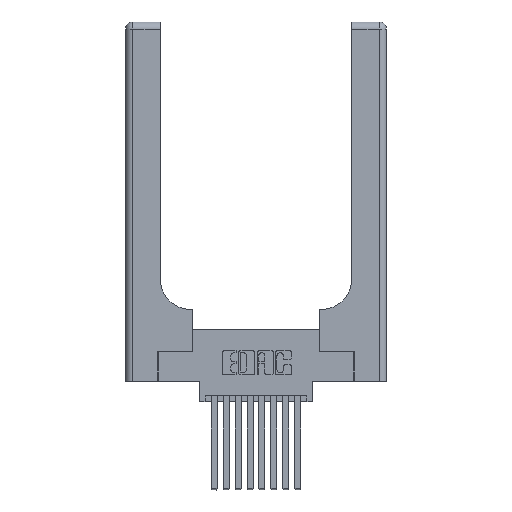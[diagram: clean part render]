
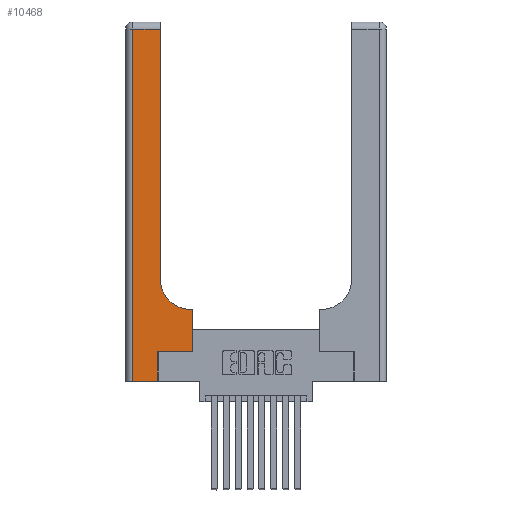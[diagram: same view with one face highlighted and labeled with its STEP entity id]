
A CAD part, top view. The second image highlights one B-rep face of the part: STEP entity #10468.
In plain terms, the highlighted planar face has unit normal (0, 0, 1).
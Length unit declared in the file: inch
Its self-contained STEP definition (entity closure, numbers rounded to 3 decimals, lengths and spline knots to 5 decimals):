
#297 = DIRECTION ( 'NONE',  ( -1., 0., 0. ) ) ;
#305 = ORIENTED_EDGE ( 'NONE', *, *, #3835, .T. ) ;
#359 = VERTEX_POINT ( 'NONE', #2186 ) ;
#690 = VECTOR ( 'NONE', #14108, 39.37008 ) ;
#743 = CARTESIAN_POINT ( 'NONE',  ( 0.06, 3., 0.37 ) ) ;
#803 = EDGE_LOOP ( 'NONE', ( #5306, #8881, #305, #12754, #1064, #12064, #5554, #12509, #13203 ) ) ;
#893 = DIRECTION ( 'NONE',  ( 0., 0., -1. ) ) ;
#1064 = ORIENTED_EDGE ( 'NONE', *, *, #12910, .T. ) ;
#1365 = VERTEX_POINT ( 'NONE', #3940 ) ;
#1384 = DIRECTION ( 'NONE',  ( 1., 0., 0. ) ) ;
#1552 = LINE ( 'NONE', #8978, #8720 ) ;
#1645 = CIRCLE ( 'NONE', #3491, 0.25 ) ;
#1737 = LINE ( 'NONE', #7882, #10046 ) ;
#1900 = DIRECTION ( 'NONE',  ( 0., 0., -1. ) ) ;
#2186 = CARTESIAN_POINT ( 'NONE',  ( 0.06, 2.94, 0.37 ) ) ;
#2346 = LINE ( 'NONE', #2623, #4280 ) ;
#2623 = CARTESIAN_POINT ( 'NONE',  ( 0., 0., 0.37 ) ) ;
#2685 = VERTEX_POINT ( 'NONE', #6079 ) ;
#2797 = FACE_OUTER_BOUND ( 'NONE', #803, .T. ) ;
#3039 = VERTEX_POINT ( 'NONE', #4269 ) ;
#3098 = LINE ( 'NONE', #8757, #5809 ) ;
#3119 = DIRECTION ( 'NONE',  ( 0., -1., 0. ) ) ;
#3139 = DIRECTION ( 'NONE',  ( -1., 0., 0. ) ) ;
#3248 = CARTESIAN_POINT ( 'NONE',  ( 0., 3., 0.37 ) ) ;
#3491 = AXIS2_PLACEMENT_3D ( 'NONE', #15745, #893, #11869 ) ;
#3690 = DIRECTION ( 'NONE',  ( -1., 0., 0. ) ) ;
#3835 = EDGE_CURVE ( 'NONE', #359, #3039, #9405, .T. ) ;
#3873 = VERTEX_POINT ( 'NONE', #9351 ) ;
#3940 = CARTESIAN_POINT ( 'NONE',  ( 0.5415, 0.6, 0.37 ) ) ;
#4109 = VERTEX_POINT ( 'NONE', #12369 ) ;
#4269 = CARTESIAN_POINT ( 'NONE',  ( 0.06, 0., 0.37 ) ) ;
#4280 = VECTOR ( 'NONE', #10075, 39.37008 ) ;
#4537 = CARTESIAN_POINT ( 'NONE',  ( 0.2915, 0.85, 0.37 ) ) ;
#4542 = EDGE_CURVE ( 'NONE', #5244, #359, #7250, .T. ) ;
#4607 = EDGE_CURVE ( 'NONE', #7030, #2685, #9582, .T. ) ;
#5244 = VERTEX_POINT ( 'NONE', #9042 ) ;
#5306 = ORIENTED_EDGE ( 'NONE', *, *, #8269, .T. ) ;
#5554 = ORIENTED_EDGE ( 'NONE', *, *, #4607, .T. ) ;
#5809 = VECTOR ( 'NONE', #1384, 39.37008 ) ;
#5884 = EDGE_CURVE ( 'NONE', #2685, #1365, #13234, .T. ) ;
#6079 = CARTESIAN_POINT ( 'NONE',  ( 0.5585, 0.6, 0.37 ) ) ;
#7030 = VERTEX_POINT ( 'NONE', #7881 ) ;
#7250 = LINE ( 'NONE', #7409, #10349 ) ;
#7313 = EDGE_CURVE ( 'NONE', #3039, #3873, #2346, .T. ) ;
#7409 = CARTESIAN_POINT ( 'NONE',  ( 0., 2.94, 0.37 ) ) ;
#7881 = CARTESIAN_POINT ( 'NONE',  ( 0.5585, 0.25, 0.37 ) ) ;
#7882 = CARTESIAN_POINT ( 'NONE',  ( 0.269, 0., 0.37 ) ) ;
#8269 = EDGE_CURVE ( 'NONE', #15666, #5244, #1552, .T. ) ;
#8720 = VECTOR ( 'NONE', #10246, 39.37008 ) ;
#8757 = CARTESIAN_POINT ( 'NONE',  ( 0.269, 0.25, 0.37 ) ) ;
#8881 = ORIENTED_EDGE ( 'NONE', *, *, #4542, .T. ) ;
#8964 = VECTOR ( 'NONE', #297, 39.37008 ) ;
#8978 = CARTESIAN_POINT ( 'NONE',  ( 0.2915, 3., 0.37 ) ) ;
#9042 = CARTESIAN_POINT ( 'NONE',  ( 0.2915, 2.94, 0.37 ) ) ;
#9351 = CARTESIAN_POINT ( 'NONE',  ( 0.269, 0., 0.37 ) ) ;
#9405 = LINE ( 'NONE', #743, #15414 ) ;
#9582 = LINE ( 'NONE', #12881, #690 ) ;
#9897 = EDGE_CURVE ( 'NONE', #1365, #15666, #1645, .T. ) ;
#10046 = VECTOR ( 'NONE', #12976, 39.37008 ) ;
#10075 = DIRECTION ( 'NONE',  ( 1., 0., 0. ) ) ;
#10246 = DIRECTION ( 'NONE',  ( 0., 1., 0. ) ) ;
#10349 = VECTOR ( 'NONE', #3690, 39.37008 ) ;
#10468 = ADVANCED_FACE ( 'NONE', ( #2797 ), #11905, .F. ) ;
#11360 = CARTESIAN_POINT ( 'NONE',  ( 0.2915, 0.6, 0.37 ) ) ;
#11869 = DIRECTION ( 'NONE',  ( 1., 0., 0. ) ) ;
#11905 = PLANE ( 'NONE',  #11989 ) ;
#11989 = AXIS2_PLACEMENT_3D ( 'NONE', #3248, #1900, #3139 ) ;
#12064 = ORIENTED_EDGE ( 'NONE', *, *, #12545, .T. ) ;
#12369 = CARTESIAN_POINT ( 'NONE',  ( 0.269, 0.25, 0.37 ) ) ;
#12509 = ORIENTED_EDGE ( 'NONE', *, *, #5884, .T. ) ;
#12545 = EDGE_CURVE ( 'NONE', #4109, #7030, #3098, .T. ) ;
#12754 = ORIENTED_EDGE ( 'NONE', *, *, #7313, .T. ) ;
#12881 = CARTESIAN_POINT ( 'NONE',  ( 0.5585, 0.25, 0.37 ) ) ;
#12910 = EDGE_CURVE ( 'NONE', #3873, #4109, #1737, .T. ) ;
#12976 = DIRECTION ( 'NONE',  ( 0., 1., 0. ) ) ;
#13203 = ORIENTED_EDGE ( 'NONE', *, *, #9897, .T. ) ;
#13234 = LINE ( 'NONE', #11360, #8964 ) ;
#14108 = DIRECTION ( 'NONE',  ( 0., 1., 0. ) ) ;
#15414 = VECTOR ( 'NONE', #3119, 39.37008 ) ;
#15666 = VERTEX_POINT ( 'NONE', #4537 ) ;
#15745 = CARTESIAN_POINT ( 'NONE',  ( 0.5415, 0.85, 0.37 ) ) ;
